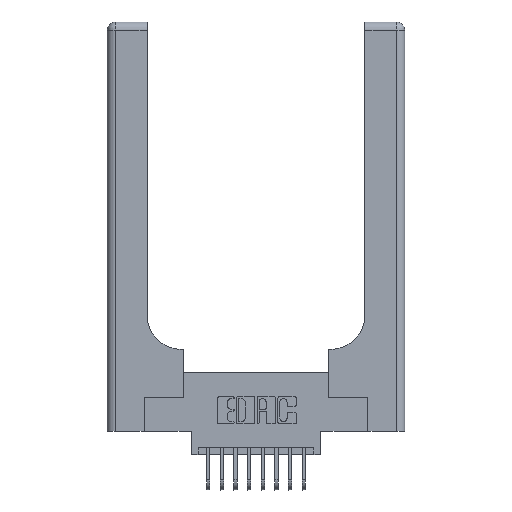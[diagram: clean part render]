
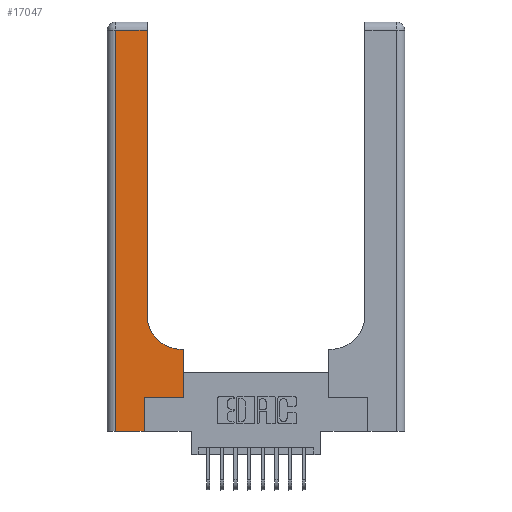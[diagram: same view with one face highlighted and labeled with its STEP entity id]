
A CAD part, top view. The second image highlights one B-rep face of the part: STEP entity #17047.
In plain terms, the highlighted planar face has unit normal (0, 0, 1).
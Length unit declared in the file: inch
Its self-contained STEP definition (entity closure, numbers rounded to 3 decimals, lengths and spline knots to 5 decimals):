
#54 = PLANE ( 'NONE',  #2483 ) ;
#817 = EDGE_CURVE ( 'NONE', #6998, #13108, #7088, .T. ) ;
#967 = VERTEX_POINT ( 'NONE', #3164 ) ;
#985 = CARTESIAN_POINT ( 'NONE',  ( 0.2915, 0.6, 0.37 ) ) ;
#1005 = LINE ( 'NONE', #8230, #12458 ) ;
#1226 = DIRECTION ( 'NONE',  ( 0., 0., -1. ) ) ;
#1333 = LINE ( 'NONE', #8969, #2417 ) ;
#1654 = VECTOR ( 'NONE', #17829, 39.37008 ) ;
#1941 = AXIS2_PLACEMENT_3D ( 'NONE', #3693, #10720, #6676 ) ;
#2417 = VECTOR ( 'NONE', #13121, 39.37008 ) ;
#2483 = AXIS2_PLACEMENT_3D ( 'NONE', #12348, #1226, #5472 ) ;
#2731 = LINE ( 'NONE', #16390, #10514 ) ;
#2936 = EDGE_CURVE ( 'NONE', #13108, #5255, #13270, .T. ) ;
#3164 = CARTESIAN_POINT ( 'NONE',  ( 0.5585, 0.6, 0.37 ) ) ;
#3693 = CARTESIAN_POINT ( 'NONE',  ( 0.5415, 0.85, 0.37 ) ) ;
#3812 = CARTESIAN_POINT ( 'NONE',  ( 0.269, 0., 0.37 ) ) ;
#4103 = CARTESIAN_POINT ( 'NONE',  ( 0.2915, 0.85, 0.37 ) ) ;
#4188 = CARTESIAN_POINT ( 'NONE',  ( 0.5415, 0.6, 0.37 ) ) ;
#4391 = ORIENTED_EDGE ( 'NONE', *, *, #16517, .T. ) ;
#4426 = DIRECTION ( 'NONE',  ( 1., 0., 0. ) ) ;
#4449 = ORIENTED_EDGE ( 'NONE', *, *, #817, .T. ) ;
#4543 = EDGE_CURVE ( 'NONE', #5255, #967, #1333, .T. ) ;
#4715 = EDGE_LOOP ( 'NONE', ( #4391, #11540, #16052, #7975, #4449, #16079, #10877, #11758, #17050 ) ) ;
#4901 = CARTESIAN_POINT ( 'NONE',  ( 0., 0., 0.37 ) ) ;
#4975 = LINE ( 'NONE', #4901, #17258 ) ;
#5174 = VECTOR ( 'NONE', #17379, 39.37008 ) ;
#5255 = VERTEX_POINT ( 'NONE', #12066 ) ;
#5472 = DIRECTION ( 'NONE',  ( -1., 0., 0. ) ) ;
#5578 = DIRECTION ( 'NONE',  ( 0., -1., 0. ) ) ;
#6676 = DIRECTION ( 'NONE',  ( 1., 0., 0. ) ) ;
#6707 = EDGE_CURVE ( 'NONE', #967, #10343, #16585, .T. ) ;
#6808 = CARTESIAN_POINT ( 'NONE',  ( 0.269, 0., 0.37 ) ) ;
#6998 = VERTEX_POINT ( 'NONE', #3812 ) ;
#7088 = LINE ( 'NONE', #6808, #1654 ) ;
#7111 = CARTESIAN_POINT ( 'NONE',  ( 0., 2.94, 0.37 ) ) ;
#7317 = EDGE_CURVE ( 'NONE', #15697, #12581, #8591, .T. ) ;
#7438 = VECTOR ( 'NONE', #4426, 39.37008 ) ;
#7702 = FACE_OUTER_BOUND ( 'NONE', #4715, .T. ) ;
#7959 = EDGE_CURVE ( 'NONE', #12581, #11757, #1005, .T. ) ;
#7975 = ORIENTED_EDGE ( 'NONE', *, *, #11932, .T. ) ;
#8230 = CARTESIAN_POINT ( 'NONE',  ( 0.06, 3., 0.37 ) ) ;
#8591 = LINE ( 'NONE', #7111, #9249 ) ;
#8712 = CARTESIAN_POINT ( 'NONE',  ( 0.2915, 2.94, 0.37 ) ) ;
#8969 = CARTESIAN_POINT ( 'NONE',  ( 0.5585, 0.25, 0.37 ) ) ;
#9249 = VECTOR ( 'NONE', #14994, 39.37008 ) ;
#10343 = VERTEX_POINT ( 'NONE', #4188 ) ;
#10418 = CIRCLE ( 'NONE', #1941, 0.25 ) ;
#10514 = VECTOR ( 'NONE', #12196, 39.37008 ) ;
#10720 = DIRECTION ( 'NONE',  ( 0., 0., -1. ) ) ;
#10877 = ORIENTED_EDGE ( 'NONE', *, *, #4543, .T. ) ;
#11315 = EDGE_CURVE ( 'NONE', #10343, #15636, #10418, .T. ) ;
#11468 = CARTESIAN_POINT ( 'NONE',  ( 0.06, 0., 0.37 ) ) ;
#11540 = ORIENTED_EDGE ( 'NONE', *, *, #7317, .T. ) ;
#11757 = VERTEX_POINT ( 'NONE', #11468 ) ;
#11758 = ORIENTED_EDGE ( 'NONE', *, *, #6707, .T. ) ;
#11863 = CARTESIAN_POINT ( 'NONE',  ( 0.269, 0.25, 0.37 ) ) ;
#11932 = EDGE_CURVE ( 'NONE', #11757, #6998, #4975, .T. ) ;
#12066 = CARTESIAN_POINT ( 'NONE',  ( 0.5585, 0.25, 0.37 ) ) ;
#12196 = DIRECTION ( 'NONE',  ( 0., 1., 0. ) ) ;
#12348 = CARTESIAN_POINT ( 'NONE',  ( 0., 3., 0.37 ) ) ;
#12458 = VECTOR ( 'NONE', #5578, 39.37008 ) ;
#12581 = VERTEX_POINT ( 'NONE', #17045 ) ;
#13108 = VERTEX_POINT ( 'NONE', #11863 ) ;
#13121 = DIRECTION ( 'NONE',  ( 0., 1., 0. ) ) ;
#13270 = LINE ( 'NONE', #14011, #7438 ) ;
#14011 = CARTESIAN_POINT ( 'NONE',  ( 0.269, 0.25, 0.37 ) ) ;
#14994 = DIRECTION ( 'NONE',  ( -1., 0., 0. ) ) ;
#15636 = VERTEX_POINT ( 'NONE', #4103 ) ;
#15697 = VERTEX_POINT ( 'NONE', #8712 ) ;
#15982 = DIRECTION ( 'NONE',  ( 1., 0., 0. ) ) ;
#16052 = ORIENTED_EDGE ( 'NONE', *, *, #7959, .T. ) ;
#16079 = ORIENTED_EDGE ( 'NONE', *, *, #2936, .T. ) ;
#16390 = CARTESIAN_POINT ( 'NONE',  ( 0.2915, 3., 0.37 ) ) ;
#16517 = EDGE_CURVE ( 'NONE', #15636, #15697, #2731, .T. ) ;
#16585 = LINE ( 'NONE', #985, #5174 ) ;
#17045 = CARTESIAN_POINT ( 'NONE',  ( 0.06, 2.94, 0.37 ) ) ;
#17047 = ADVANCED_FACE ( 'NONE', ( #7702 ), #54, .F. ) ;
#17050 = ORIENTED_EDGE ( 'NONE', *, *, #11315, .T. ) ;
#17258 = VECTOR ( 'NONE', #15982, 39.37008 ) ;
#17379 = DIRECTION ( 'NONE',  ( -1., 0., 0. ) ) ;
#17829 = DIRECTION ( 'NONE',  ( 0., 1., 0. ) ) ;
